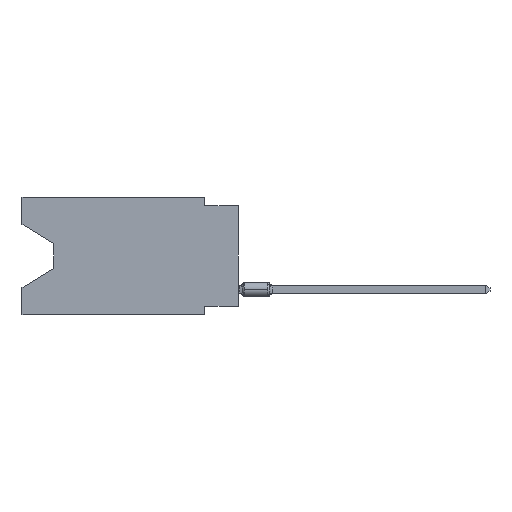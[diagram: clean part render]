
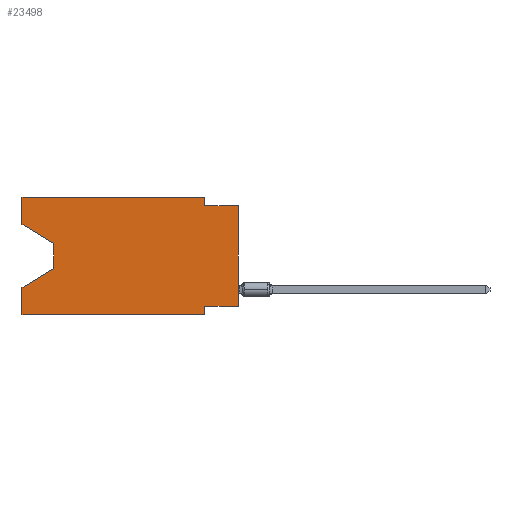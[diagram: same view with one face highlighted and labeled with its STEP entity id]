
A CAD part, left-side view. The second image highlights one B-rep face of the part: STEP entity #23498.
In plain terms, the highlighted planar face has unit normal (-1, 0, 0).
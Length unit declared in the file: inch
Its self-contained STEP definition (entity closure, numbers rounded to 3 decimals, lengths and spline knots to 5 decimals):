
#98 = CARTESIAN_POINT ( 'NONE',  ( 0., 0.645, 0. ) ) ;
#685 = ORIENTED_EDGE ( 'NONE', *, *, #6984, .F. ) ;
#809 = VERTEX_POINT ( 'NONE', #14109 ) ;
#1285 = ORIENTED_EDGE ( 'NONE', *, *, #24016, .T. ) ;
#1410 = VERTEX_POINT ( 'NONE', #20204 ) ;
#1466 = DIRECTION ( 'NONE',  ( 0., 0., 1. ) ) ;
#1805 = ORIENTED_EDGE ( 'NONE', *, *, #21937, .T. ) ;
#2011 = PLANE ( 'NONE',  #14672 ) ;
#2138 = CARTESIAN_POINT ( 'NONE',  ( 0., 0.645, 0. ) ) ;
#2482 = ORIENTED_EDGE ( 'NONE', *, *, #15752, .F. ) ;
#2504 = CARTESIAN_POINT ( 'NONE',  ( 0., 0., -0.025 ) ) ;
#2942 = VECTOR ( 'NONE', #20162, 39.37008 ) ;
#3178 = VERTEX_POINT ( 'NONE', #23169 ) ;
#3230 = LINE ( 'NONE', #18255, #5684 ) ;
#3290 = LINE ( 'NONE', #10826, #24127 ) ;
#3551 = LINE ( 'NONE', #98, #10049 ) ;
#3622 = DIRECTION ( 'NONE',  ( 0., 0., -1. ) ) ;
#4148 = LINE ( 'NONE', #21131, #16212 ) ;
#4516 = LINE ( 'NONE', #13874, #17852 ) ;
#4739 = ORIENTED_EDGE ( 'NONE', *, *, #15717, .F. ) ;
#4949 = CARTESIAN_POINT ( 'NONE',  ( 0., 0.55, -0.138 ) ) ;
#5052 = VERTEX_POINT ( 'NONE', #15020 ) ;
#5160 = ORIENTED_EDGE ( 'NONE', *, *, #5608, .T. ) ;
#5608 = EDGE_CURVE ( 'NONE', #809, #5868, #4148, .T. ) ;
#5684 = VECTOR ( 'NONE', #10527, 39.37008 ) ;
#5868 = VERTEX_POINT ( 'NONE', #4949 ) ;
#5932 = LINE ( 'NONE', #9644, #22935 ) ;
#6306 = CARTESIAN_POINT ( 'NONE',  ( 0., 0.55, -0.212 ) ) ;
#6809 = VERTEX_POINT ( 'NONE', #9415 ) ;
#6945 = CARTESIAN_POINT ( 'NONE',  ( 0., 0.645, 0. ) ) ;
#6984 = EDGE_CURVE ( 'NONE', #20624, #22026, #12357, .T. ) ;
#7030 = EDGE_LOOP ( 'NONE', ( #5160, #1805, #1285, #2482, #14781, #15485, #4739, #9713, #685, #10134, #10095, #17872 ) ) ;
#7371 = DIRECTION ( 'NONE',  ( 0., 0., 1. ) ) ;
#7387 = LINE ( 'NONE', #16492, #10295 ) ;
#7460 = DIRECTION ( 'NONE',  ( 1., 0., 0. ) ) ;
#7502 = CARTESIAN_POINT ( 'NONE',  ( 0., 0., -0.325 ) ) ;
#7832 = VECTOR ( 'NONE', #9323, 39.37008 ) ;
#8163 = DIRECTION ( 'NONE',  ( 0., 0.855, -0.519 ) ) ;
#9026 = CARTESIAN_POINT ( 'NONE',  ( 0., 0.1, -0.025 ) ) ;
#9276 = CARTESIAN_POINT ( 'NONE',  ( 0., 0.645, -0.35 ) ) ;
#9304 = VECTOR ( 'NONE', #10395, 39.37008 ) ;
#9323 = DIRECTION ( 'NONE',  ( 0., 0., -1. ) ) ;
#9362 = EDGE_CURVE ( 'NONE', #22668, #3178, #4516, .T. ) ;
#9415 = CARTESIAN_POINT ( 'NONE',  ( 0., 0.1, -0.35 ) ) ;
#9472 = LINE ( 'NONE', #16735, #20765 ) ;
#9644 = CARTESIAN_POINT ( 'NONE',  ( 0., 0.1, -0.35 ) ) ;
#9713 = ORIENTED_EDGE ( 'NONE', *, *, #19273, .T. ) ;
#9883 = LINE ( 'NONE', #6306, #17450 ) ;
#10049 = VECTOR ( 'NONE', #1466, 39.37008 ) ;
#10095 = ORIENTED_EDGE ( 'NONE', *, *, #9362, .F. ) ;
#10134 = ORIENTED_EDGE ( 'NONE', *, *, #16930, .F. ) ;
#10295 = VECTOR ( 'NONE', #19930, 39.37008 ) ;
#10395 = DIRECTION ( 'NONE',  ( 0., -1., 0. ) ) ;
#10448 = EDGE_CURVE ( 'NONE', #809, #22668, #3290, .T. ) ;
#10527 = DIRECTION ( 'NONE',  ( 0., -1., 0. ) ) ;
#10826 = CARTESIAN_POINT ( 'NONE',  ( 0., 0.645, 0. ) ) ;
#11201 = EDGE_CURVE ( 'NONE', #12374, #6809, #3230, .T. ) ;
#11547 = DIRECTION ( 'NONE',  ( 0., -0.855, -0.519 ) ) ;
#12357 = LINE ( 'NONE', #2504, #9304 ) ;
#12374 = VERTEX_POINT ( 'NONE', #9276 ) ;
#12598 = EDGE_CURVE ( 'NONE', #15676, #6809, #5932, .T. ) ;
#12802 = CARTESIAN_POINT ( 'NONE',  ( 0., 0.1, -0.325 ) ) ;
#13115 = FACE_OUTER_BOUND ( 'NONE', #7030, .T. ) ;
#13874 = CARTESIAN_POINT ( 'NONE',  ( 0., 0.645, 0. ) ) ;
#14109 = CARTESIAN_POINT ( 'NONE',  ( 0., 0.645, -0.08025 ) ) ;
#14672 = AXIS2_PLACEMENT_3D ( 'NONE', #2138, #7460, #3622 ) ;
#14781 = ORIENTED_EDGE ( 'NONE', *, *, #11201, .T. ) ;
#15020 = CARTESIAN_POINT ( 'NONE',  ( 0., 0.645, -0.26975 ) ) ;
#15292 = DIRECTION ( 'NONE',  ( 0., 0., -1. ) ) ;
#15485 = ORIENTED_EDGE ( 'NONE', *, *, #12598, .F. ) ;
#15676 = VERTEX_POINT ( 'NONE', #12802 ) ;
#15717 = EDGE_CURVE ( 'NONE', #21274, #15676, #24217, .T. ) ;
#15752 = EDGE_CURVE ( 'NONE', #12374, #5052, #3551, .T. ) ;
#16212 = VECTOR ( 'NONE', #11547, 39.37008 ) ;
#16492 = CARTESIAN_POINT ( 'NONE',  ( 0., 0., 0. ) ) ;
#16735 = CARTESIAN_POINT ( 'NONE',  ( 0., 0.1, 0. ) ) ;
#16930 = EDGE_CURVE ( 'NONE', #3178, #20624, #9472, .T. ) ;
#17280 = CARTESIAN_POINT ( 'NONE',  ( 0., 0., -0.325 ) ) ;
#17450 = VECTOR ( 'NONE', #8163, 39.37008 ) ;
#17852 = VECTOR ( 'NONE', #23074, 39.37008 ) ;
#17872 = ORIENTED_EDGE ( 'NONE', *, *, #10448, .F. ) ;
#18255 = CARTESIAN_POINT ( 'NONE',  ( 0., 0.645, -0.35 ) ) ;
#18663 = CARTESIAN_POINT ( 'NONE',  ( 0., 0.55, -0.138 ) ) ;
#19273 = EDGE_CURVE ( 'NONE', #21274, #22026, #7387, .T. ) ;
#19519 = CARTESIAN_POINT ( 'NONE',  ( 0., 0., -0.025 ) ) ;
#19930 = DIRECTION ( 'NONE',  ( 0., 0., 1. ) ) ;
#20162 = DIRECTION ( 'NONE',  ( 0., 1., 0. ) ) ;
#20204 = CARTESIAN_POINT ( 'NONE',  ( 0., 0.55, -0.212 ) ) ;
#20624 = VERTEX_POINT ( 'NONE', #9026 ) ;
#20765 = VECTOR ( 'NONE', #24222, 39.37008 ) ;
#21131 = CARTESIAN_POINT ( 'NONE',  ( 0., 0.645, -0.08025 ) ) ;
#21274 = VERTEX_POINT ( 'NONE', #17280 ) ;
#21937 = EDGE_CURVE ( 'NONE', #5868, #1410, #22466, .T. ) ;
#22026 = VERTEX_POINT ( 'NONE', #19519 ) ;
#22466 = LINE ( 'NONE', #18663, #7832 ) ;
#22668 = VERTEX_POINT ( 'NONE', #6945 ) ;
#22935 = VECTOR ( 'NONE', #15292, 39.37008 ) ;
#23074 = DIRECTION ( 'NONE',  ( 0., -1., 0. ) ) ;
#23169 = CARTESIAN_POINT ( 'NONE',  ( 0., 0.1, 0. ) ) ;
#23498 = ADVANCED_FACE ( 'NONE', ( #13115 ), #2011, .F. ) ;
#24016 = EDGE_CURVE ( 'NONE', #1410, #5052, #9883, .T. ) ;
#24127 = VECTOR ( 'NONE', #7371, 39.37008 ) ;
#24217 = LINE ( 'NONE', #7502, #2942 ) ;
#24222 = DIRECTION ( 'NONE',  ( 0., 0., -1. ) ) ;
